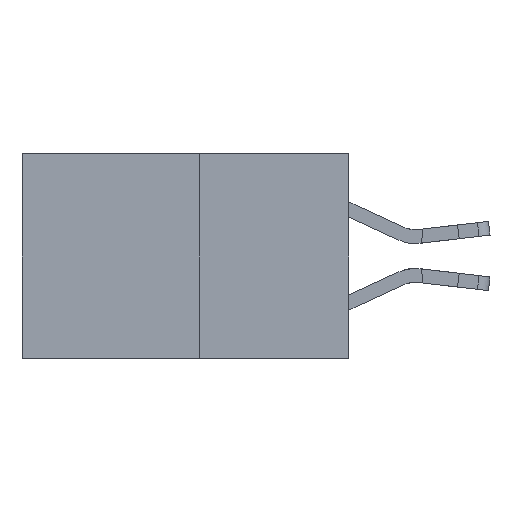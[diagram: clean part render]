
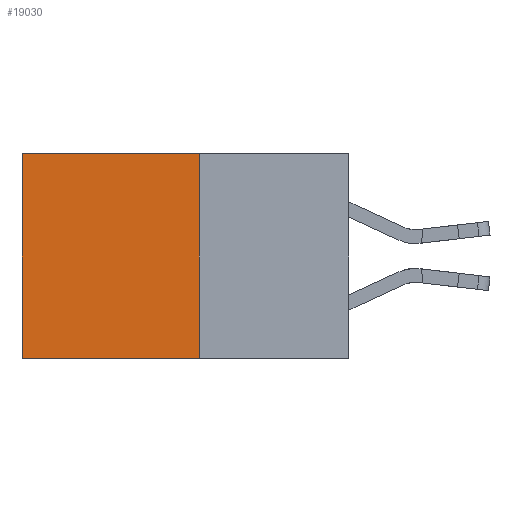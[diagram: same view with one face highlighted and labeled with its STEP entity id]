
A CAD part, left-side view. The second image highlights one B-rep face of the part: STEP entity #19030.
In plain terms, the highlighted planar face has unit normal (-1, 0, 0).
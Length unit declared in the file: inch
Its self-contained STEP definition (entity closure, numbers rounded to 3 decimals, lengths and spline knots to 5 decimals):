
#287 = DIRECTION ( 'NONE',  ( 0., 1., 0. ) ) ;
#1667 = VERTEX_POINT ( 'NONE', #3402 ) ;
#2747 = ORIENTED_EDGE ( 'NONE', *, *, #11585, .F. ) ;
#3000 = CARTESIAN_POINT ( 'NONE',  ( 0.277, 0.27, -0.37 ) ) ;
#3060 = VERTEX_POINT ( 'NONE', #9405 ) ;
#3402 = CARTESIAN_POINT ( 'NONE',  ( 0.277, 0.27, -0.37 ) ) ;
#3506 = LINE ( 'NONE', #15695, #19039 ) ;
#3906 = DIRECTION ( 'NONE',  ( 0., 0., -1. ) ) ;
#4202 = VECTOR ( 'NONE', #3906, 39.37008 ) ;
#4528 = EDGE_CURVE ( 'NONE', #17311, #3060, #11177, .T. ) ;
#5129 = DIRECTION ( 'NONE',  ( 0., 0., -1. ) ) ;
#5807 = CARTESIAN_POINT ( 'NONE',  ( 0.277, 0.27, 0. ) ) ;
#7215 = DIRECTION ( 'NONE',  ( 0., 0., -1. ) ) ;
#7239 = CARTESIAN_POINT ( 'NONE',  ( 0.277, 0.59, -0.37 ) ) ;
#7700 = ORIENTED_EDGE ( 'NONE', *, *, #17240, .T. ) ;
#9405 = CARTESIAN_POINT ( 'NONE',  ( 0.277, 0.59, 0. ) ) ;
#10363 = CARTESIAN_POINT ( 'NONE',  ( 0.277, 0.59, -0.37 ) ) ;
#10386 = DIRECTION ( 'NONE',  ( 0., 1., 0. ) ) ;
#11177 = LINE ( 'NONE', #5807, #26179 ) ;
#11585 = EDGE_CURVE ( 'NONE', #17311, #1667, #3506, .T. ) ;
#12625 = EDGE_LOOP ( 'NONE', ( #7700, #13196, #2747, #13188 ) ) ;
#13188 = ORIENTED_EDGE ( 'NONE', *, *, #4528, .T. ) ;
#13196 = ORIENTED_EDGE ( 'NONE', *, *, #23409, .F. ) ;
#14971 = VECTOR ( 'NONE', #10386, 39.37008 ) ;
#15695 = CARTESIAN_POINT ( 'NONE',  ( 0.277, 0.27, -0.37 ) ) ;
#17240 = EDGE_CURVE ( 'NONE', #3060, #17638, #20994, .T. ) ;
#17311 = VERTEX_POINT ( 'NONE', #22593 ) ;
#17638 = VERTEX_POINT ( 'NONE', #7239 ) ;
#17815 = DIRECTION ( 'NONE',  ( 1., 0., 0. ) ) ;
#19030 = ADVANCED_FACE ( 'NONE', ( #26492 ), #25786, .F. ) ;
#19039 = VECTOR ( 'NONE', #7215, 39.37008 ) ;
#20994 = LINE ( 'NONE', #10363, #4202 ) ;
#21099 = LINE ( 'NONE', #22675, #14971 ) ;
#22593 = CARTESIAN_POINT ( 'NONE',  ( 0.277, 0.27, 0. ) ) ;
#22675 = CARTESIAN_POINT ( 'NONE',  ( 0.277, 0.27, -0.37 ) ) ;
#23409 = EDGE_CURVE ( 'NONE', #1667, #17638, #21099, .T. ) ;
#25786 = PLANE ( 'NONE',  #26525 ) ;
#26179 = VECTOR ( 'NONE', #287, 39.37008 ) ;
#26492 = FACE_OUTER_BOUND ( 'NONE', #12625, .T. ) ;
#26525 = AXIS2_PLACEMENT_3D ( 'NONE', #3000, #17815, #5129 ) ;
